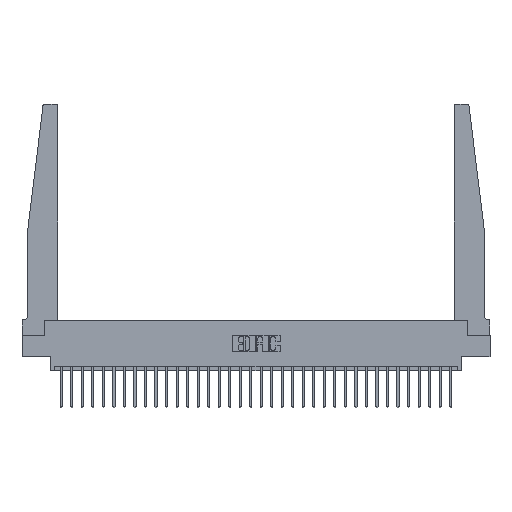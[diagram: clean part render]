
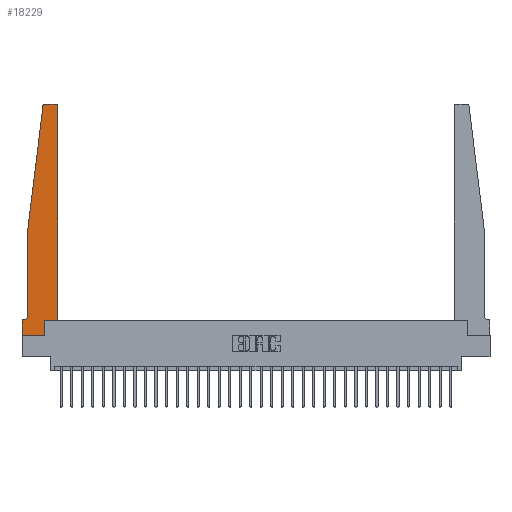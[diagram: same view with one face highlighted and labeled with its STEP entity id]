
A CAD part, top view. The second image highlights one B-rep face of the part: STEP entity #18229.
In plain terms, the highlighted planar face has unit normal (0, 0, 1).
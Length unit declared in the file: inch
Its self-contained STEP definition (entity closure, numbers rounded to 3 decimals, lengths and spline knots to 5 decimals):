
#791 = VECTOR ( 'NONE', #23198, 39.37008 ) ;
#846 = CARTESIAN_POINT ( 'NONE',  ( 0.25, 2.75, 0.37 ) ) ;
#1205 = DIRECTION ( 'NONE',  ( 1., 0., 0. ) ) ;
#1222 = AXIS2_PLACEMENT_3D ( 'NONE', #18368, #10876, #1527 ) ;
#1527 = DIRECTION ( 'NONE',  ( 1., 0., 0. ) ) ;
#1530 = DIRECTION ( 'NONE',  ( 1., 0., 0. ) ) ;
#2447 = LINE ( 'NONE', #11969, #17105 ) ;
#2756 = LINE ( 'NONE', #28690, #12953 ) ;
#2875 = LINE ( 'NONE', #846, #24911 ) ;
#3248 = EDGE_CURVE ( 'NONE', #8308, #25803, #8399, .T. ) ;
#3585 = EDGE_CURVE ( 'NONE', #3695, #8308, #11656, .T. ) ;
#3634 = ORIENTED_EDGE ( 'NONE', *, *, #20126, .T. ) ;
#3695 = VERTEX_POINT ( 'NONE', #8194 ) ;
#3873 = CARTESIAN_POINT ( 'NONE',  ( 0., 0.1875, 0.37 ) ) ;
#3915 = VERTEX_POINT ( 'NONE', #15053 ) ;
#4077 = VECTOR ( 'NONE', #18347, 39.37008 ) ;
#4297 = LINE ( 'NONE', #10572, #4077 ) ;
#4366 = VERTEX_POINT ( 'NONE', #17550 ) ;
#5580 = CARTESIAN_POINT ( 'NONE',  ( 0.395, 2.72, 0.37 ) ) ;
#5686 = EDGE_CURVE ( 'NONE', #13572, #20629, #23187, .T. ) ;
#5750 = DIRECTION ( 'NONE',  ( 1., 0., 0. ) ) ;
#5816 = CARTESIAN_POINT ( 'NONE',  ( 0.065, 1.25, 0.37 ) ) ;
#6202 = FACE_OUTER_BOUND ( 'NONE', #16566, .T. ) ;
#6329 = LINE ( 'NONE', #27446, #23868 ) ;
#6720 = ORIENTED_EDGE ( 'NONE', *, *, #3248, .T. ) ;
#8194 = CARTESIAN_POINT ( 'NONE',  ( 0.27653, 2.75, 0.37 ) ) ;
#8308 = VERTEX_POINT ( 'NONE', #9151 ) ;
#8384 = PLANE ( 'NONE',  #28158 ) ;
#8399 = LINE ( 'NONE', #27339, #20668 ) ;
#8643 = ORIENTED_EDGE ( 'NONE', *, *, #21871, .T. ) ;
#9037 = VECTOR ( 'NONE', #28208, 39.37008 ) ;
#9078 = EDGE_CURVE ( 'NONE', #14282, #30221, #29303, .T. ) ;
#9151 = CARTESIAN_POINT ( 'NONE',  ( 0.24675, 2.72367, 0.37 ) ) ;
#9603 = CARTESIAN_POINT ( 'NONE',  ( 0.425, 0.18, 0.37 ) ) ;
#9671 = EDGE_CURVE ( 'NONE', #25803, #14282, #27394, .T. ) ;
#9895 = ORIENTED_EDGE ( 'NONE', *, *, #15200, .T. ) ;
#10572 = CARTESIAN_POINT ( 'NONE',  ( 0., 0., 0.37 ) ) ;
#10829 = CARTESIAN_POINT ( 'NONE',  ( 0.2605, 0., 0.37 ) ) ;
#10876 = DIRECTION ( 'NONE',  ( 0., 0., 1. ) ) ;
#11459 = CARTESIAN_POINT ( 'NONE',  ( 0.065, 1.25, 0.37 ) ) ;
#11638 = CARTESIAN_POINT ( 'NONE',  ( 0., 0., 0.37 ) ) ;
#11656 = CIRCLE ( 'NONE', #1222, 0.03 ) ;
#11836 = CARTESIAN_POINT ( 'NONE',  ( 0.425, 2.72, 0.37 ) ) ;
#11969 = CARTESIAN_POINT ( 'NONE',  ( 0.2605, 0.18, 0.37 ) ) ;
#12899 = DIRECTION ( 'NONE',  ( -1., 0., 0. ) ) ;
#12953 = VECTOR ( 'NONE', #28852, 39.37008 ) ;
#13148 = VERTEX_POINT ( 'NONE', #10829 ) ;
#13511 = DIRECTION ( 'NONE',  ( 0., 0., -1. ) ) ;
#13572 = VERTEX_POINT ( 'NONE', #11836 ) ;
#13728 = LINE ( 'NONE', #16644, #791 ) ;
#14282 = VERTEX_POINT ( 'NONE', #24014 ) ;
#15053 = CARTESIAN_POINT ( 'NONE',  ( 0.2605, 0.18, 0.37 ) ) ;
#15200 = EDGE_CURVE ( 'NONE', #20798, #13572, #13728, .T. ) ;
#15226 = DIRECTION ( 'NONE',  ( 0., 1., 0. ) ) ;
#15252 = LINE ( 'NONE', #27041, #29012 ) ;
#15529 = DIRECTION ( 'NONE',  ( 0., 0., 1. ) ) ;
#16566 = EDGE_LOOP ( 'NONE', ( #3634, #23937, #6720, #23076, #16894, #8643, #21617, #26893, #28432, #29903, #9895, #30049 ) ) ;
#16644 = CARTESIAN_POINT ( 'NONE',  ( 0.425, 0.18, 0.37 ) ) ;
#16894 = ORIENTED_EDGE ( 'NONE', *, *, #9078, .T. ) ;
#16939 = AXIS2_PLACEMENT_3D ( 'NONE', #27608, #13511, #12899 ) ;
#17105 = VECTOR ( 'NONE', #15226, 39.37008 ) ;
#17550 = CARTESIAN_POINT ( 'NONE',  ( 0., 0.1875, 0.37 ) ) ;
#18229 = ADVANCED_FACE ( 'NONE', ( #6202 ), #8384, .T. ) ;
#18238 = VERTEX_POINT ( 'NONE', #11638 ) ;
#18347 = DIRECTION ( 'NONE',  ( 0., -1., 0. ) ) ;
#18368 = CARTESIAN_POINT ( 'NONE',  ( 0.27653, 2.72, 0.37 ) ) ;
#19785 = CARTESIAN_POINT ( 'NONE',  ( 0.395, 2.75, 0.37 ) ) ;
#20126 = EDGE_CURVE ( 'NONE', #20629, #3695, #2875, .T. ) ;
#20629 = VERTEX_POINT ( 'NONE', #19785 ) ;
#20668 = VECTOR ( 'NONE', #26743, 39.37008 ) ;
#20707 = AXIS2_PLACEMENT_3D ( 'NONE', #5580, #15529, #1205 ) ;
#20798 = VERTEX_POINT ( 'NONE', #9603 ) ;
#21617 = ORIENTED_EDGE ( 'NONE', *, *, #23447, .T. ) ;
#21871 = EDGE_CURVE ( 'NONE', #30221, #4366, #2756, .T. ) ;
#22209 = EDGE_CURVE ( 'NONE', #3915, #20798, #6329, .T. ) ;
#22865 = DIRECTION ( 'NONE',  ( 0., 0., 1. ) ) ;
#23076 = ORIENTED_EDGE ( 'NONE', *, *, #9671, .T. ) ;
#23187 = CIRCLE ( 'NONE', #20707, 0.03 ) ;
#23198 = DIRECTION ( 'NONE',  ( 0., 1., 0. ) ) ;
#23447 = EDGE_CURVE ( 'NONE', #4366, #18238, #4297, .T. ) ;
#23868 = VECTOR ( 'NONE', #27914, 39.37008 ) ;
#23937 = ORIENTED_EDGE ( 'NONE', *, *, #3585, .T. ) ;
#24014 = CARTESIAN_POINT ( 'NONE',  ( 0.065, 0.2375, 0.37 ) ) ;
#24553 = CARTESIAN_POINT ( 'NONE',  ( 0.015, 0.1875, 0.37 ) ) ;
#24911 = VECTOR ( 'NONE', #26658, 39.37008 ) ;
#25803 = VERTEX_POINT ( 'NONE', #5816 ) ;
#26658 = DIRECTION ( 'NONE',  ( -1., 0., 0. ) ) ;
#26721 = EDGE_CURVE ( 'NONE', #18238, #13148, #15252, .T. ) ;
#26743 = DIRECTION ( 'NONE',  ( -0.122, -0.992, 0. ) ) ;
#26893 = ORIENTED_EDGE ( 'NONE', *, *, #26721, .T. ) ;
#27041 = CARTESIAN_POINT ( 'NONE',  ( 0., 0., 0.37 ) ) ;
#27339 = CARTESIAN_POINT ( 'NONE',  ( 0.065, 1.25, 0.37 ) ) ;
#27394 = LINE ( 'NONE', #11459, #9037 ) ;
#27446 = CARTESIAN_POINT ( 'NONE',  ( 0.425, 0.18, 0.37 ) ) ;
#27608 = CARTESIAN_POINT ( 'NONE',  ( 0.015, 0.2375, 0.37 ) ) ;
#27914 = DIRECTION ( 'NONE',  ( 1., 0., 0. ) ) ;
#28158 = AXIS2_PLACEMENT_3D ( 'NONE', #3873, #22865, #1530 ) ;
#28208 = DIRECTION ( 'NONE',  ( 0., -1., 0. ) ) ;
#28432 = ORIENTED_EDGE ( 'NONE', *, *, #28549, .T. ) ;
#28549 = EDGE_CURVE ( 'NONE', #13148, #3915, #2447, .T. ) ;
#28690 = CARTESIAN_POINT ( 'NONE',  ( 0.065, 0.1875, 0.37 ) ) ;
#28852 = DIRECTION ( 'NONE',  ( -1., 0., 0. ) ) ;
#29012 = VECTOR ( 'NONE', #5750, 39.37008 ) ;
#29303 = CIRCLE ( 'NONE', #16939, 0.05 ) ;
#29903 = ORIENTED_EDGE ( 'NONE', *, *, #22209, .T. ) ;
#30049 = ORIENTED_EDGE ( 'NONE', *, *, #5686, .T. ) ;
#30221 = VERTEX_POINT ( 'NONE', #24553 ) ;
